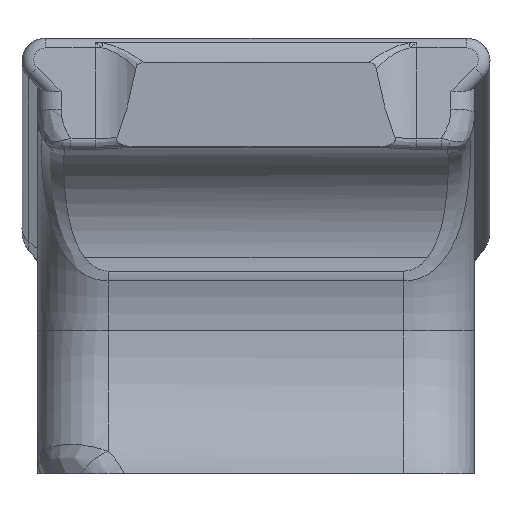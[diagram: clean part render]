
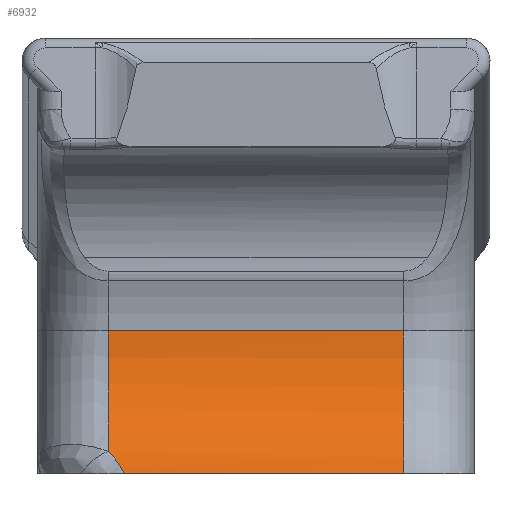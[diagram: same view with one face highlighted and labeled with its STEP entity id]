
A CAD part, left-side view. The second image highlights one B-rep face of the part: STEP entity #6932.
In plain terms, the highlighted cylindrical face has radius 14.287 mm (diameter 28.575 mm), a partial arc.
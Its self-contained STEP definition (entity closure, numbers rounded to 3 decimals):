
#80 = VERTEX_POINT ( 'NONE', #4931 ) ;
#221 = EDGE_LOOP ( 'NONE', ( #1141, #1179, #1415, #1483, #1599 ) ) ;
#461 = VERTEX_POINT ( 'NONE', #6864 ) ;
#726 = VECTOR ( 'NONE', #1717, 1000. ) ;
#758 = LINE ( 'NONE', #8062, #726 ) ;
#773 = DIRECTION ( 'NONE',  ( 0., 1., 0. ) ) ;
#801 = DIRECTION ( 'NONE',  ( 1., 0., 0. ) ) ;
#1141 = ORIENTED_EDGE ( 'NONE', *, *, #8035, .T. ) ;
#1152 = CARTESIAN_POINT ( 'NONE',  ( 76.653, -72.447, -1.367 ) ) ;
#1179 = ORIENTED_EDGE ( 'NONE', *, *, #7414, .T. ) ;
#1415 = ORIENTED_EDGE ( 'NONE', *, *, #1683, .T. ) ;
#1483 = ORIENTED_EDGE ( 'NONE', *, *, #3466, .T. ) ;
#1599 = ORIENTED_EDGE ( 'NONE', *, *, #4501, .T. ) ;
#1683 = EDGE_CURVE ( 'NONE', #7215, #80, #6597, .T. ) ;
#1717 = DIRECTION ( 'NONE',  ( 0., 1., 0. ) ) ;
#1855 = DIRECTION ( 'NONE',  ( 0., -1., 0. ) ) ;
#1887 = CARTESIAN_POINT ( 'NONE',  ( 84.171, -70.726, -13.516 ) ) ;
#1905 = CARTESIAN_POINT ( 'NONE',  ( 84.171, -72.447, -13.516 ) ) ;
#2028 = AXIS2_PLACEMENT_3D ( 'NONE', #2255, #2127, #2154 ) ;
#2127 = DIRECTION ( 'NONE',  ( 0., 1., 0. ) ) ;
#2142 = CIRCLE ( 'NONE', #5731, 14.288 ) ;
#2154 = DIRECTION ( 'NONE',  ( 1., 0., 0. ) ) ;
#2255 = CARTESIAN_POINT ( 'NONE',  ( 76.653, -45.593, -1.367 ) ) ;
#2827 = CARTESIAN_POINT ( 'NONE',  ( 90.94, -45.593, -1.367 ) ) ;
#3137 = CARTESIAN_POINT ( 'NONE',  ( 85.556, -46.401, -12.541 ) ) ;
#3194 = CARTESIAN_POINT ( 'NONE',  ( 85.595, -46.379, -12.51 ) ) ;
#3466 = EDGE_CURVE ( 'NONE', #80, #461, #7316, .T. ) ;
#3573 = DIRECTION ( 'NONE',  ( 0., -1., 0. ) ) ;
#3708 = CARTESIAN_POINT ( 'NONE',  ( 85.113, -46.642, -12.89 ) ) ;
#4254 = VERTEX_POINT ( 'NONE', #8366 ) ;
#4352 = CARTESIAN_POINT ( 'NONE',  ( 84.171, -46.951, -13.516 ) ) ;
#4479 = AXIS2_PLACEMENT_3D ( 'NONE', #1152, #773, #801 ) ;
#4501 = EDGE_CURVE ( 'NONE', #461, #7307, #6871, .T. ) ;
#4931 = CARTESIAN_POINT ( 'NONE',  ( 86.612, -45.593, -11.611 ) ) ;
#5039 = CARTESIAN_POINT ( 'NONE',  ( 85.529, -46.415, -12.562 ) ) ;
#5046 = CARTESIAN_POINT ( 'NONE',  ( 85.685, -46.326, -12.437 ) ) ;
#5731 = AXIS2_PLACEMENT_3D ( 'NONE', #7388, #3573, #8014 ) ;
#6128 = CARTESIAN_POINT ( 'NONE',  ( 84.671, -46.816, -13.206 ) ) ;
#6597 = CIRCLE ( 'NONE', #2028, 14.288 ) ;
#6702 = FACE_OUTER_BOUND ( 'NONE', #221, .T. ) ;
#6800 = VECTOR ( 'NONE', #1855, 1000. ) ;
#6864 = CARTESIAN_POINT ( 'NONE',  ( 84.171, -46.951, -13.516 ) ) ;
#6871 = LINE ( 'NONE', #1905, #6800 ) ;
#6932 = ADVANCED_FACE ( 'NONE', ( #6702 ), #8057, .F. ) ;
#7215 = VERTEX_POINT ( 'NONE', #2827 ) ;
#7307 = VERTEX_POINT ( 'NONE', #1887 ) ;
#7316 = B_SPLINE_CURVE_WITH_KNOTS ( 'NONE', 3,
 ( #7357, #7415, #8111, #8234, #8286, #8263, #5046, #3194, #3137, #5039, #8165, #3708, #6128, #4352 ),
 .UNSPECIFIED., .F., .F.,
 ( 4, 2, 2, 1, 1, 2, 2, 4 ),
 ( 0., 0.25, 0.375, 0.437, 0.469, 0.484, 0.5, 1. ),
 .UNSPECIFIED. ) ;
#7357 = CARTESIAN_POINT ( 'NONE',  ( 86.612, -45.593, -11.611 ) ) ;
#7388 = CARTESIAN_POINT ( 'NONE',  ( 76.653, -70.726, -1.367 ) ) ;
#7414 = EDGE_CURVE ( 'NONE', #4254, #7215, #758, .T. ) ;
#7415 = CARTESIAN_POINT ( 'NONE',  ( 86.453, -45.756, -11.766 ) ) ;
#8014 = DIRECTION ( 'NONE',  ( 1., 0., 0. ) ) ;
#8035 = EDGE_CURVE ( 'NONE', #7307, #4254, #2142, .T. ) ;
#8057 = CYLINDRICAL_SURFACE ( 'NONE', #4479, 14.288 ) ;
#8062 = CARTESIAN_POINT ( 'NONE',  ( 90.94, -72.447, -1.367 ) ) ;
#8111 = CARTESIAN_POINT ( 'NONE',  ( 86.281, -45.908, -11.925 ) ) ;
#8165 = CARTESIAN_POINT ( 'NONE',  ( 85.515, -46.423, -12.573 ) ) ;
#8234 = CARTESIAN_POINT ( 'NONE',  ( 86.005, -46.117, -12.169 ) ) ;
#8263 = CARTESIAN_POINT ( 'NONE',  ( 85.761, -46.28, -12.375 ) ) ;
#8286 = CARTESIAN_POINT ( 'NONE',  ( 85.909, -46.184, -12.251 ) ) ;
#8366 = CARTESIAN_POINT ( 'NONE',  ( 90.94, -70.726, -1.367 ) ) ;
